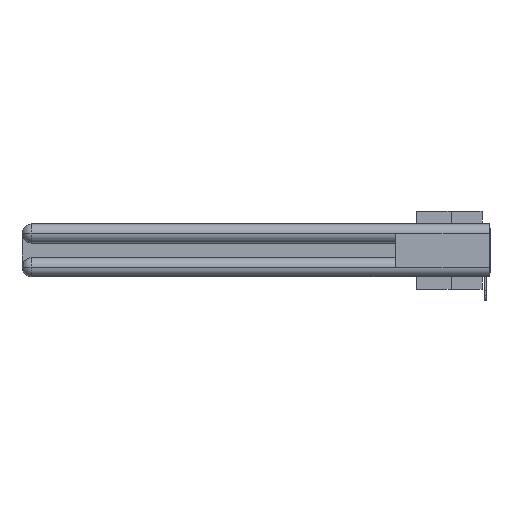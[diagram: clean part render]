
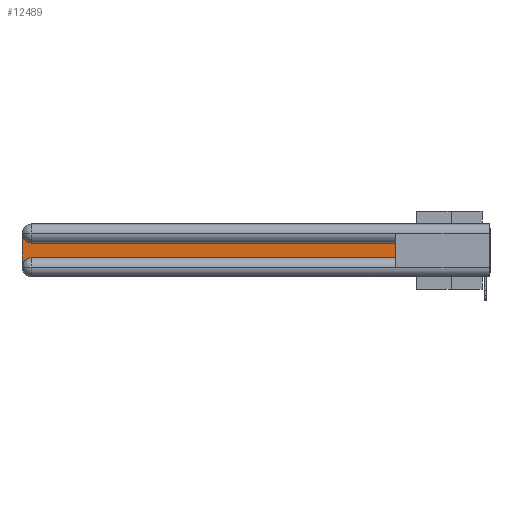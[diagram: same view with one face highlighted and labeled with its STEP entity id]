
A CAD part, left-side view. The second image highlights one B-rep face of the part: STEP entity #12489.
In plain terms, the highlighted planar face has unit normal (-1, 0, 0).
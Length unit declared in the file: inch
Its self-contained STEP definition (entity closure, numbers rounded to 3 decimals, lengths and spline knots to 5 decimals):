
#683 = ORIENTED_EDGE ( 'NONE', *, *, #29089, .T. ) ;
#2128 = VERTEX_POINT ( 'NONE', #29475 ) ;
#2783 = EDGE_CURVE ( 'NONE', #24349, #14940, #3423, .T. ) ;
#3423 = CIRCLE ( 'NONE', #22872, 0.06 ) ;
#3889 = EDGE_CURVE ( 'NONE', #29942, #27192, #28202, .T. ) ;
#4230 = VECTOR ( 'NONE', #23603, 39.37008 ) ;
#5716 = CARTESIAN_POINT ( 'NONE',  ( 0.075, 2.94, -0.2175 ) ) ;
#6504 = CARTESIAN_POINT ( 'NONE',  ( 0.075, 0.6, -0.1225 ) ) ;
#7000 = DIRECTION ( 'NONE',  ( 1., 0., 0. ) ) ;
#8021 = VECTOR ( 'NONE', #9219, 39.37008 ) ;
#8059 = ORIENTED_EDGE ( 'NONE', *, *, #14927, .T. ) ;
#9219 = DIRECTION ( 'NONE',  ( 0., 1., 0. ) ) ;
#9243 = DIRECTION ( 'NONE',  ( 0., 0., -1. ) ) ;
#9270 = CARTESIAN_POINT ( 'NONE',  ( 0.075, 0.6, -0.2175 ) ) ;
#10331 = AXIS2_PLACEMENT_3D ( 'NONE', #15718, #22907, #18278 ) ;
#11345 = PLANE ( 'NONE',  #29483 ) ;
#11829 = CARTESIAN_POINT ( 'NONE',  ( 0.075, 3., -0.1225 ) ) ;
#11847 = DIRECTION ( 'NONE',  ( 1., 0., 0. ) ) ;
#12489 = ADVANCED_FACE ( 'NONE', ( #23638 ), #11345, .F. ) ;
#14401 = DIRECTION ( 'NONE',  ( 0., 0., -1. ) ) ;
#14927 = EDGE_CURVE ( 'NONE', #27192, #22927, #29589, .T. ) ;
#14940 = VERTEX_POINT ( 'NONE', #17637 ) ;
#15718 = CARTESIAN_POINT ( 'NONE',  ( 0.075, 2.94, -0.2775 ) ) ;
#15784 = CARTESIAN_POINT ( 'NONE',  ( 0.075, 0.6, -0.2175 ) ) ;
#16648 = CARTESIAN_POINT ( 'NONE',  ( 0.075, 3., -0.2175 ) ) ;
#17637 = CARTESIAN_POINT ( 'NONE',  ( 0.075, 3., -0.0625 ) ) ;
#18216 = VECTOR ( 'NONE', #19863, 39.37008 ) ;
#18278 = DIRECTION ( 'NONE',  ( 0., 0., -1. ) ) ;
#18640 = EDGE_CURVE ( 'NONE', #14940, #29942, #21916, .T. ) ;
#19338 = VECTOR ( 'NONE', #26382, 39.37008 ) ;
#19434 = ORIENTED_EDGE ( 'NONE', *, *, #2783, .T. ) ;
#19722 = ORIENTED_EDGE ( 'NONE', *, *, #18640, .T. ) ;
#19863 = DIRECTION ( 'NONE',  ( 0., -1., 0. ) ) ;
#20001 = EDGE_LOOP ( 'NONE', ( #683, #19434, #19722, #31026, #8059, #22523 ) ) ;
#21916 = LINE ( 'NONE', #16648, #19338 ) ;
#22523 = ORIENTED_EDGE ( 'NONE', *, *, #24787, .T. ) ;
#22872 = AXIS2_PLACEMENT_3D ( 'NONE', #31433, #11847, #14401 ) ;
#22907 = DIRECTION ( 'NONE',  ( 1., 0., 0. ) ) ;
#22927 = VERTEX_POINT ( 'NONE', #9270 ) ;
#23603 = DIRECTION ( 'NONE',  ( 0., 0., 1. ) ) ;
#23638 = FACE_OUTER_BOUND ( 'NONE', #20001, .T. ) ;
#24349 = VERTEX_POINT ( 'NONE', #27003 ) ;
#24787 = EDGE_CURVE ( 'NONE', #22927, #2128, #31519, .T. ) ;
#25687 = LINE ( 'NONE', #6504, #8021 ) ;
#26206 = CARTESIAN_POINT ( 'NONE',  ( 0.075, 3., -0.2775 ) ) ;
#26382 = DIRECTION ( 'NONE',  ( 0., 0., -1. ) ) ;
#27003 = CARTESIAN_POINT ( 'NONE',  ( 0.075, 2.94, -0.1225 ) ) ;
#27192 = VERTEX_POINT ( 'NONE', #5716 ) ;
#28202 = CIRCLE ( 'NONE', #10331, 0.06 ) ;
#29089 = EDGE_CURVE ( 'NONE', #2128, #24349, #25687, .T. ) ;
#29475 = CARTESIAN_POINT ( 'NONE',  ( 0.075, 0.6, -0.1225 ) ) ;
#29483 = AXIS2_PLACEMENT_3D ( 'NONE', #11829, #7000, #9243 ) ;
#29589 = LINE ( 'NONE', #29744, #18216 ) ;
#29744 = CARTESIAN_POINT ( 'NONE',  ( 0.075, 0.6, -0.2175 ) ) ;
#29942 = VERTEX_POINT ( 'NONE', #26206 ) ;
#31026 = ORIENTED_EDGE ( 'NONE', *, *, #3889, .T. ) ;
#31433 = CARTESIAN_POINT ( 'NONE',  ( 0.075, 2.94, -0.0625 ) ) ;
#31519 = LINE ( 'NONE', #15784, #4230 ) ;
